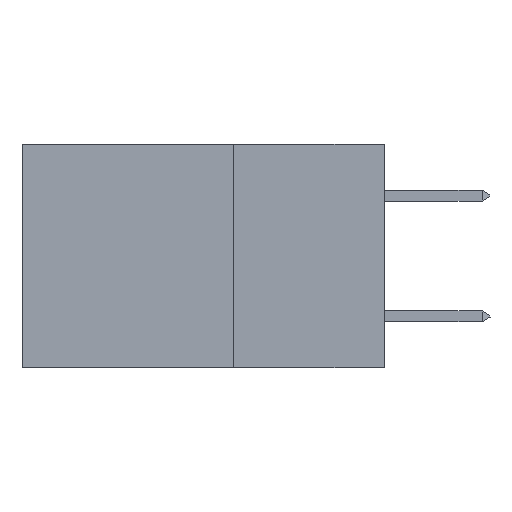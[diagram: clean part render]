
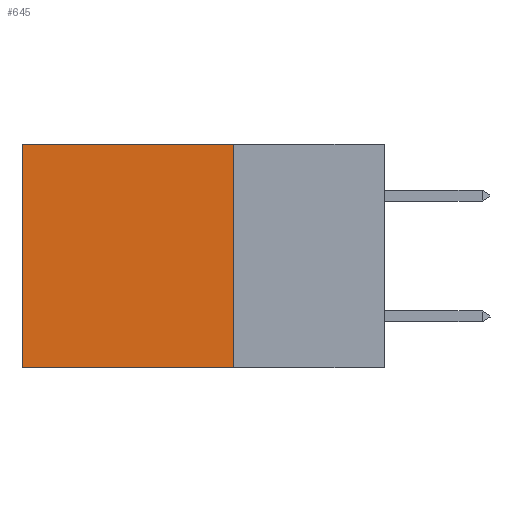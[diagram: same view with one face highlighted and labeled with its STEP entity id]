
A CAD part, left-side view. The second image highlights one B-rep face of the part: STEP entity #645.
In plain terms, the highlighted planar face has unit normal (-1, 0, 0).
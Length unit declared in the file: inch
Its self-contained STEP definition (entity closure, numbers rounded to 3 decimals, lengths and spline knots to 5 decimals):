
#104 = DIRECTION ( 'NONE',  ( 0., 1., 0. ) ) ;
#645 = ADVANCED_FACE ( 'NONE', ( #16861 ), #21021, .F. ) ;
#1217 = DIRECTION ( 'NONE',  ( 0., 0., -1. ) ) ;
#1385 = VECTOR ( 'NONE', #104, 39.37008 ) ;
#1967 = ORIENTED_EDGE ( 'NONE', *, *, #20352, .F. ) ;
#4340 = ORIENTED_EDGE ( 'NONE', *, *, #14470, .T. ) ;
#5286 = CARTESIAN_POINT ( 'NONE',  ( 0.2875, 0.25, -0.37 ) ) ;
#5418 = CARTESIAN_POINT ( 'NONE',  ( 0.2875, 0.25, -0.37 ) ) ;
#6044 = ORIENTED_EDGE ( 'NONE', *, *, #26307, .T. ) ;
#8234 = EDGE_LOOP ( 'NONE', ( #6044, #1967, #19226, #4340 ) ) ;
#9086 = VECTOR ( 'NONE', #27523, 39.37008 ) ;
#9593 = EDGE_CURVE ( 'NONE', #17111, #12655, #22629, .T. ) ;
#10166 = VECTOR ( 'NONE', #16443, 39.37008 ) ;
#10639 = CARTESIAN_POINT ( 'NONE',  ( 0.2875, 0.6, 0. ) ) ;
#12220 = CARTESIAN_POINT ( 'NONE',  ( 0.2875, 0.25, 0. ) ) ;
#12655 = VERTEX_POINT ( 'NONE', #5286 ) ;
#12842 = CARTESIAN_POINT ( 'NONE',  ( 0.2875, 0.25, 0. ) ) ;
#13617 = LINE ( 'NONE', #18162, #20486 ) ;
#14470 = EDGE_CURVE ( 'NONE', #17111, #16493, #18951, .T. ) ;
#15660 = CARTESIAN_POINT ( 'NONE',  ( 0.2875, 0.6, -0.37 ) ) ;
#15920 = VERTEX_POINT ( 'NONE', #15660 ) ;
#16231 = AXIS2_PLACEMENT_3D ( 'NONE', #23310, #23209, #1217 ) ;
#16443 = DIRECTION ( 'NONE',  ( 0., 0., -1. ) ) ;
#16493 = VERTEX_POINT ( 'NONE', #10639 ) ;
#16861 = FACE_OUTER_BOUND ( 'NONE', #8234, .T. ) ;
#17111 = VERTEX_POINT ( 'NONE', #12842 ) ;
#18093 = LINE ( 'NONE', #5418, #9086 ) ;
#18162 = CARTESIAN_POINT ( 'NONE',  ( 0.2875, 0.6, 0. ) ) ;
#18951 = LINE ( 'NONE', #26882, #1385 ) ;
#19226 = ORIENTED_EDGE ( 'NONE', *, *, #9593, .F. ) ;
#20352 = EDGE_CURVE ( 'NONE', #12655, #15920, #18093, .T. ) ;
#20486 = VECTOR ( 'NONE', #25127, 39.37008 ) ;
#21021 = PLANE ( 'NONE',  #16231 ) ;
#22629 = LINE ( 'NONE', #12220, #10166 ) ;
#23209 = DIRECTION ( 'NONE',  ( 1., 0., 0. ) ) ;
#23310 = CARTESIAN_POINT ( 'NONE',  ( 0.2875, 0.25, 0. ) ) ;
#25127 = DIRECTION ( 'NONE',  ( 0., 0., -1. ) ) ;
#26307 = EDGE_CURVE ( 'NONE', #16493, #15920, #13617, .T. ) ;
#26882 = CARTESIAN_POINT ( 'NONE',  ( 0.2875, 0.25, 0. ) ) ;
#27523 = DIRECTION ( 'NONE',  ( 0., 1., 0. ) ) ;
